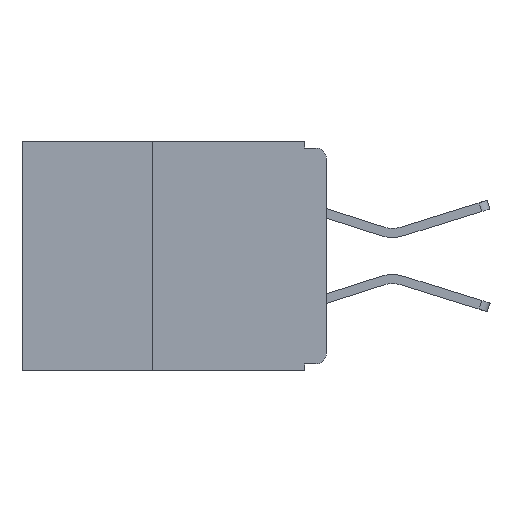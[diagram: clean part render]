
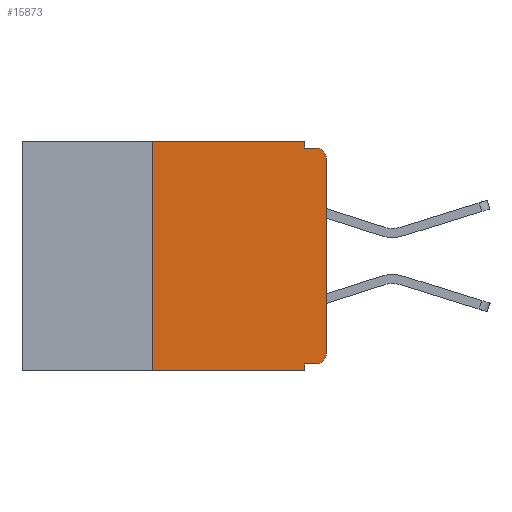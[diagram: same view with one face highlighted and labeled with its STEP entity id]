
A CAD part, left-side view. The second image highlights one B-rep face of the part: STEP entity #15873.
In plain terms, the highlighted planar face has unit normal (-1, 0, 0).
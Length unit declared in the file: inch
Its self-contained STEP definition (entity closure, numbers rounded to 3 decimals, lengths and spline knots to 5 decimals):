
#293 = CARTESIAN_POINT ( 'NONE',  ( 0., 0.031, -0.33 ) ) ;
#314 = LINE ( 'NONE', #11003, #4124 ) ;
#556 = EDGE_CURVE ( 'NONE', #15940, #6472, #314, .T. ) ;
#579 = LINE ( 'NONE', #18011, #16406 ) ;
#1059 = CARTESIAN_POINT ( 'NONE',  ( 0., 0., 0. ) ) ;
#1338 = EDGE_CURVE ( 'NONE', #11035, #13768, #4355, .T. ) ;
#1442 = VERTEX_POINT ( 'NONE', #9298 ) ;
#1445 = CIRCLE ( 'NONE', #8234, 0.015 ) ;
#1542 = EDGE_CURVE ( 'NONE', #1442, #15940, #12229, .T. ) ;
#1651 = LINE ( 'NONE', #1059, #9029 ) ;
#1865 = DIRECTION ( 'NONE',  ( 1., 0., 0. ) ) ;
#2373 = VECTOR ( 'NONE', #4594, 39.37008 ) ;
#2897 = CARTESIAN_POINT ( 'NONE',  ( 0., 0.015, -0.025 ) ) ;
#3134 = DIRECTION ( 'NONE',  ( -1., 0., 0. ) ) ;
#3344 = CARTESIAN_POINT ( 'NONE',  ( 0., 0., -0.32 ) ) ;
#3372 = DIRECTION ( 'NONE',  ( 0., 0., -1. ) ) ;
#3726 = EDGE_CURVE ( 'NONE', #6472, #6840, #11448, .T. ) ;
#4124 = VECTOR ( 'NONE', #14935, 39.37008 ) ;
#4355 = CIRCLE ( 'NONE', #13531, 0.015 ) ;
#4594 = DIRECTION ( 'NONE',  ( 0., 1., 0. ) ) ;
#4754 = CARTESIAN_POINT ( 'NONE',  ( 0., 0.031, 0. ) ) ;
#4793 = CARTESIAN_POINT ( 'NONE',  ( 0., 0., -0.305 ) ) ;
#5530 = AXIS2_PLACEMENT_3D ( 'NONE', #14105, #1865, #12682 ) ;
#5637 = EDGE_CURVE ( 'NONE', #17459, #7353, #14125, .T. ) ;
#5772 = CARTESIAN_POINT ( 'NONE',  ( 0., 0.015, -0.305 ) ) ;
#6472 = VERTEX_POINT ( 'NONE', #4754 ) ;
#6530 = VECTOR ( 'NONE', #15579, 39.37008 ) ;
#6608 = DIRECTION ( 'NONE',  ( 0., -1., 0. ) ) ;
#6840 = VERTEX_POINT ( 'NONE', #19379 ) ;
#6853 = VERTEX_POINT ( 'NONE', #293 ) ;
#7009 = LINE ( 'NONE', #15827, #6530 ) ;
#7335 = DIRECTION ( 'NONE',  ( 0., 0., -1. ) ) ;
#7339 = EDGE_CURVE ( 'NONE', #6840, #13768, #7009, .T. ) ;
#7353 = VERTEX_POINT ( 'NONE', #15704 ) ;
#8165 = PLANE ( 'NONE',  #5530 ) ;
#8234 = AXIS2_PLACEMENT_3D ( 'NONE', #5772, #16240, #7335 ) ;
#8239 = VECTOR ( 'NONE', #13210, 39.37008 ) ;
#8358 = CARTESIAN_POINT ( 'NONE',  ( 0., 0.25, 0. ) ) ;
#9029 = VECTOR ( 'NONE', #16376, 39.37008 ) ;
#9298 = CARTESIAN_POINT ( 'NONE',  ( 0., 0.25, -0.33 ) ) ;
#9739 = ORIENTED_EDGE ( 'NONE', *, *, #5637, .F. ) ;
#9789 = ORIENTED_EDGE ( 'NONE', *, *, #14106, .T. ) ;
#10224 = ORIENTED_EDGE ( 'NONE', *, *, #16256, .F. ) ;
#11003 = CARTESIAN_POINT ( 'NONE',  ( 0., 0.437, 0. ) ) ;
#11035 = VERTEX_POINT ( 'NONE', #13855 ) ;
#11448 = LINE ( 'NONE', #14966, #14900 ) ;
#11556 = VECTOR ( 'NONE', #6608, 39.37008 ) ;
#12229 = LINE ( 'NONE', #17803, #8239 ) ;
#12490 = LINE ( 'NONE', #18618, #11556 ) ;
#12547 = CARTESIAN_POINT ( 'NONE',  ( 0., 0.015, -0.01 ) ) ;
#12682 = DIRECTION ( 'NONE',  ( 0., 0., -1. ) ) ;
#13210 = DIRECTION ( 'NONE',  ( 0., 0., 1. ) ) ;
#13531 = AXIS2_PLACEMENT_3D ( 'NONE', #2897, #3134, #3372 ) ;
#13768 = VERTEX_POINT ( 'NONE', #12547 ) ;
#13855 = CARTESIAN_POINT ( 'NONE',  ( 0., 0., -0.025 ) ) ;
#14105 = CARTESIAN_POINT ( 'NONE',  ( 0., 0.437, 0. ) ) ;
#14106 = EDGE_CURVE ( 'NONE', #17459, #18703, #1445, .T. ) ;
#14125 = LINE ( 'NONE', #3344, #2373 ) ;
#14899 = DIRECTION ( 'NONE',  ( 0., 0., -1. ) ) ;
#14900 = VECTOR ( 'NONE', #14899, 39.37008 ) ;
#14935 = DIRECTION ( 'NONE',  ( 0., -1., 0. ) ) ;
#14966 = CARTESIAN_POINT ( 'NONE',  ( 0., 0.031, 0. ) ) ;
#14977 = EDGE_CURVE ( 'NONE', #18703, #11035, #1651, .T. ) ;
#15134 = CARTESIAN_POINT ( 'NONE',  ( 0., 0.015, -0.32 ) ) ;
#15579 = DIRECTION ( 'NONE',  ( 0., -1., 0. ) ) ;
#15704 = CARTESIAN_POINT ( 'NONE',  ( 0., 0.031, -0.32 ) ) ;
#15827 = CARTESIAN_POINT ( 'NONE',  ( 0., 0., -0.01 ) ) ;
#15873 = ADVANCED_FACE ( 'NONE', ( #15961 ), #8165, .F. ) ;
#15940 = VERTEX_POINT ( 'NONE', #8358 ) ;
#15961 = FACE_OUTER_BOUND ( 'NONE', #18624, .T. ) ;
#16240 = DIRECTION ( 'NONE',  ( -1., 0., 0. ) ) ;
#16256 = EDGE_CURVE ( 'NONE', #7353, #6853, #579, .T. ) ;
#16376 = DIRECTION ( 'NONE',  ( 0., 0., 1. ) ) ;
#16406 = VECTOR ( 'NONE', #19527, 39.37008 ) ;
#17459 = VERTEX_POINT ( 'NONE', #15134 ) ;
#17803 = CARTESIAN_POINT ( 'NONE',  ( 0., 0.25, -0.33 ) ) ;
#18011 = CARTESIAN_POINT ( 'NONE',  ( 0., 0.031, -0.33 ) ) ;
#18094 = ORIENTED_EDGE ( 'NONE', *, *, #14977, .T. ) ;
#18224 = ORIENTED_EDGE ( 'NONE', *, *, #1338, .T. ) ;
#18329 = ORIENTED_EDGE ( 'NONE', *, *, #7339, .F. ) ;
#18380 = ORIENTED_EDGE ( 'NONE', *, *, #3726, .F. ) ;
#18447 = ORIENTED_EDGE ( 'NONE', *, *, #556, .F. ) ;
#18618 = CARTESIAN_POINT ( 'NONE',  ( 0., 0.437, -0.33 ) ) ;
#18624 = EDGE_LOOP ( 'NONE', ( #18094, #18224, #18329, #18380, #18447, #18628, #18733, #10224, #9739, #9789 ) ) ;
#18628 = ORIENTED_EDGE ( 'NONE', *, *, #1542, .F. ) ;
#18703 = VERTEX_POINT ( 'NONE', #4793 ) ;
#18733 = ORIENTED_EDGE ( 'NONE', *, *, #19327, .T. ) ;
#19327 = EDGE_CURVE ( 'NONE', #1442, #6853, #12490, .T. ) ;
#19379 = CARTESIAN_POINT ( 'NONE',  ( 0., 0.031, -0.01 ) ) ;
#19527 = DIRECTION ( 'NONE',  ( 0., 0., -1. ) ) ;
